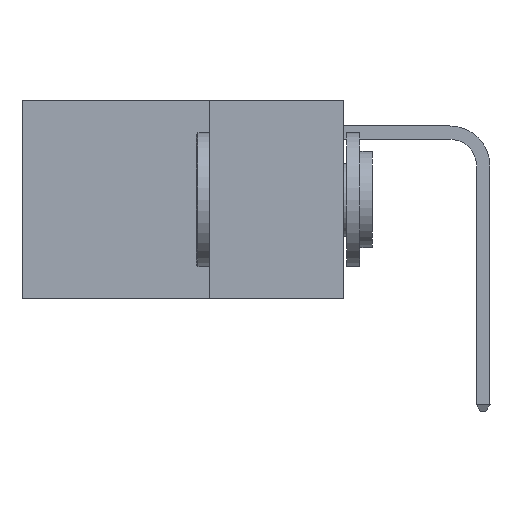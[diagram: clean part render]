
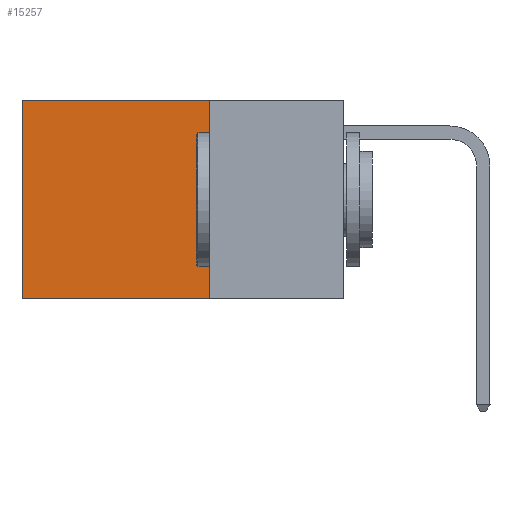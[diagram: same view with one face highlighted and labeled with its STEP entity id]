
A CAD part, left-side view. The second image highlights one B-rep face of the part: STEP entity #15257.
In plain terms, the highlighted planar face has unit normal (-1, 0, 0).
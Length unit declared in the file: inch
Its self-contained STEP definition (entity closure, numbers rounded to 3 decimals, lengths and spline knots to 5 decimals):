
#238 = VERTEX_POINT ( 'NONE', #11373 ) ;
#315 = PLANE ( 'NONE',  #14747 ) ;
#2288 = EDGE_CURVE ( 'NONE', #11273, #17724, #15816, .T. ) ;
#2455 = ORIENTED_EDGE ( 'NONE', *, *, #17592, .T. ) ;
#2464 = EDGE_CURVE ( 'NONE', #238, #17724, #28455, .T. ) ;
#4839 = ORIENTED_EDGE ( 'NONE', *, *, #6973, .F. ) ;
#4867 = DIRECTION ( 'NONE',  ( 1., 0., 0. ) ) ;
#6055 = LINE ( 'NONE', #6919, #17297 ) ;
#6919 = CARTESIAN_POINT ( 'NONE',  ( 0.2625, 0.25, 0. ) ) ;
#6947 = CARTESIAN_POINT ( 'NONE',  ( 0.2625, 0.25, 0. ) ) ;
#6973 = EDGE_CURVE ( 'NONE', #11696, #238, #11054, .T. ) ;
#9216 = DIRECTION ( 'NONE',  ( 0., 0., -1. ) ) ;
#9640 = DIRECTION ( 'NONE',  ( 0., 1., 0. ) ) ;
#9881 = VECTOR ( 'NONE', #13975, 39.37008 ) ;
#9905 = CARTESIAN_POINT ( 'NONE',  ( 0.2625, 0.25, -0.37 ) ) ;
#10441 = ORIENTED_EDGE ( 'NONE', *, *, #2464, .F. ) ;
#11054 = LINE ( 'NONE', #6947, #27910 ) ;
#11160 = FACE_OUTER_BOUND ( 'NONE', #15792, .T. ) ;
#11273 = VERTEX_POINT ( 'NONE', #14201 ) ;
#11373 = CARTESIAN_POINT ( 'NONE',  ( 0.2625, 0.25, -0.37 ) ) ;
#11696 = VERTEX_POINT ( 'NONE', #26964 ) ;
#13975 = DIRECTION ( 'NONE',  ( 0., 0., -1. ) ) ;
#14111 = CARTESIAN_POINT ( 'NONE',  ( 0.2625, 0.6, 0. ) ) ;
#14201 = CARTESIAN_POINT ( 'NONE',  ( 0.2625, 0.6, 0. ) ) ;
#14747 = AXIS2_PLACEMENT_3D ( 'NONE', #22684, #4867, #20591 ) ;
#15257 = ADVANCED_FACE ( 'NONE', ( #11160 ), #315, .F. ) ;
#15792 = EDGE_LOOP ( 'NONE', ( #20974, #10441, #4839, #2455 ) ) ;
#15816 = LINE ( 'NONE', #14111, #9881 ) ;
#17297 = VECTOR ( 'NONE', #24731, 39.37008 ) ;
#17592 = EDGE_CURVE ( 'NONE', #11696, #11273, #6055, .T. ) ;
#17724 = VERTEX_POINT ( 'NONE', #27242 ) ;
#20591 = DIRECTION ( 'NONE',  ( 0., 0., -1. ) ) ;
#20974 = ORIENTED_EDGE ( 'NONE', *, *, #2288, .T. ) ;
#22113 = VECTOR ( 'NONE', #9640, 39.37008 ) ;
#22684 = CARTESIAN_POINT ( 'NONE',  ( 0.2625, 0.25, 0. ) ) ;
#24731 = DIRECTION ( 'NONE',  ( 0., 1., 0. ) ) ;
#26964 = CARTESIAN_POINT ( 'NONE',  ( 0.2625, 0.25, 0. ) ) ;
#27242 = CARTESIAN_POINT ( 'NONE',  ( 0.2625, 0.6, -0.37 ) ) ;
#27910 = VECTOR ( 'NONE', #9216, 39.37008 ) ;
#28455 = LINE ( 'NONE', #9905, #22113 ) ;
